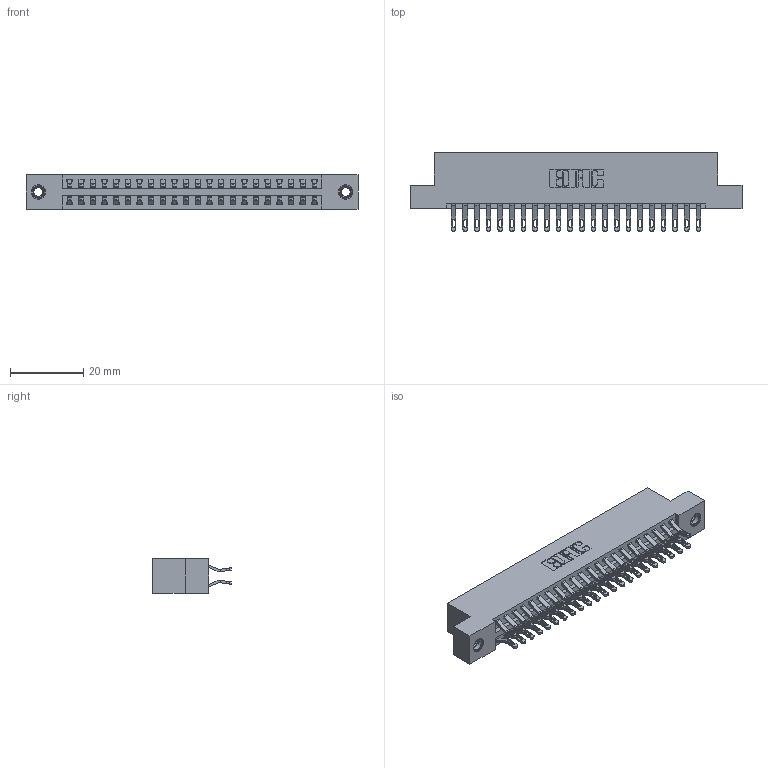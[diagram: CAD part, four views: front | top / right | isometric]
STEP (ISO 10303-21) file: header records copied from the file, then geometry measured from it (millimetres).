
FILE_DESCRIPTION (( 'STEP AP203' ), '1' );
FILE_NAME ('346-044-555-207.STEP', '2022-05-20T07:37:05', ( '' ), ( '' ), 'SwSTEP 2.0', 'SolidWorks 2020', '' );
FILE_SCHEMA (( 'CONFIG_CONTROL_DESIGN' ));
Length unit declared in the file: inch
Products named in the file (4): 345-292-001_555 Tail; 346-044-555-207; 346 Part_Flush Mounting Lugs - 0.156 Dia-TI; 345-250-001_345-250-005-103
Assembly tree (47 placements, depth 2):
  346-044-555-207
    346 Part_Flush Mounting Lugs - 0.156 Dia-TI
    345-292-001_555 Tail  x44
    345-250-001_345-250-005-103  x2
Bounding box: 90.42 x 21.46 x 9.4 mm (x, y, z)
Volume: 8776.2 mm3; surface area: 12237.9 mm2
Topology: 47 solids, 47 shells, 2734 faces, 8517 edges, 5670 vertices
Faces by surface type: plane 1560, cylinder 1158, cone 12, torus 4
Entity records: 18562 total; most frequent: CARTESIAN_POINT 3105, ORIENTED_EDGE 3002, DIRECTION 2783, EDGE_CURVE 1501, VECTOR 1241, LINE 1241, VERTEX_POINT 996, AXIS2_PLACEMENT_3D 771
